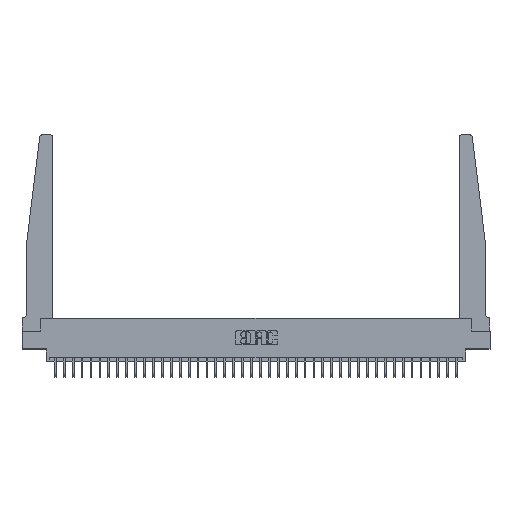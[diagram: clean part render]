
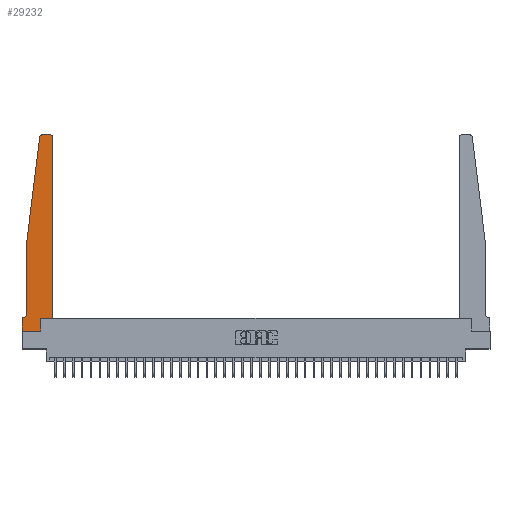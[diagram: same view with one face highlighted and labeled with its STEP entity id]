
A CAD part, top view. The second image highlights one B-rep face of the part: STEP entity #29232.
In plain terms, the highlighted planar face has unit normal (0, 0, 1).
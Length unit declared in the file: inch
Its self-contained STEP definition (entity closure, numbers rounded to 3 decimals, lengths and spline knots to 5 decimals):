
#158 = VECTOR ( 'NONE', #11250, 39.37008 ) ;
#385 = LINE ( 'NONE', #22990, #17930 ) ;
#425 = VERTEX_POINT ( 'NONE', #16666 ) ;
#760 = DIRECTION ( 'NONE',  ( 1., 0., 0. ) ) ;
#777 = CARTESIAN_POINT ( 'NONE',  ( 0.27653, 2.75, 0.37 ) ) ;
#1232 = CARTESIAN_POINT ( 'NONE',  ( 0.425, 2.72, 0.37 ) ) ;
#1611 = DIRECTION ( 'NONE',  ( -1., 0., 0. ) ) ;
#2733 = LINE ( 'NONE', #17054, #158 ) ;
#2762 = VERTEX_POINT ( 'NONE', #23885 ) ;
#2818 = VERTEX_POINT ( 'NONE', #35410 ) ;
#3502 = VECTOR ( 'NONE', #29156, 39.37008 ) ;
#5674 = CARTESIAN_POINT ( 'NONE',  ( 0.425, 0.18, 0.37 ) ) ;
#5698 = CIRCLE ( 'NONE', #6887, 0.05 ) ;
#6228 = EDGE_CURVE ( 'NONE', #24817, #22424, #14608, .T. ) ;
#6242 = EDGE_CURVE ( 'NONE', #9802, #425, #25441, .T. ) ;
#6554 = CARTESIAN_POINT ( 'NONE',  ( 0.25, 2.75, 0.37 ) ) ;
#6887 = AXIS2_PLACEMENT_3D ( 'NONE', #10128, #27002, #1611 ) ;
#7701 = CIRCLE ( 'NONE', #30194, 0.03 ) ;
#7858 = CARTESIAN_POINT ( 'NONE',  ( 0.065, 1.25, 0.37 ) ) ;
#8149 = CARTESIAN_POINT ( 'NONE',  ( 0.2605, 0.18, 0.37 ) ) ;
#8686 = DIRECTION ( 'NONE',  ( 0., 0., 1. ) ) ;
#8942 = ORIENTED_EDGE ( 'NONE', *, *, #28609, .T. ) ;
#9554 = EDGE_CURVE ( 'NONE', #26657, #9802, #35755, .T. ) ;
#9802 = VERTEX_POINT ( 'NONE', #22740 ) ;
#10128 = CARTESIAN_POINT ( 'NONE',  ( 0.015, 0.2375, 0.37 ) ) ;
#11250 = DIRECTION ( 'NONE',  ( 1., 0., 0. ) ) ;
#11584 = EDGE_CURVE ( 'NONE', #14837, #26657, #5698, .T. ) ;
#11778 = DIRECTION ( 'NONE',  ( 0., 1., 0. ) ) ;
#12047 = ORIENTED_EDGE ( 'NONE', *, *, #30227, .T. ) ;
#12601 = EDGE_CURVE ( 'NONE', #25482, #14789, #22620, .T. ) ;
#13620 = CARTESIAN_POINT ( 'NONE',  ( 0.065, 0.2375, 0.37 ) ) ;
#13943 = DIRECTION ( 'NONE',  ( 0., 0., 1. ) ) ;
#14157 = CARTESIAN_POINT ( 'NONE',  ( 0., 0., 0.37 ) ) ;
#14608 = CIRCLE ( 'NONE', #29384, 0.03 ) ;
#14747 = LINE ( 'NONE', #5674, #16177 ) ;
#14789 = VERTEX_POINT ( 'NONE', #7858 ) ;
#14837 = VERTEX_POINT ( 'NONE', #13620 ) ;
#14908 = VECTOR ( 'NONE', #34289, 39.37008 ) ;
#15116 = CARTESIAN_POINT ( 'NONE',  ( 0.395, 2.72, 0.37 ) ) ;
#15720 = CARTESIAN_POINT ( 'NONE',  ( 0.065, 0.1875, 0.37 ) ) ;
#16177 = VECTOR ( 'NONE', #11778, 39.37008 ) ;
#16666 = CARTESIAN_POINT ( 'NONE',  ( 0., 0., 0.37 ) ) ;
#17054 = CARTESIAN_POINT ( 'NONE',  ( 0.425, 0.18, 0.37 ) ) ;
#17352 = EDGE_CURVE ( 'NONE', #22424, #32955, #20651, .T. ) ;
#17930 = VECTOR ( 'NONE', #760, 39.37008 ) ;
#18146 = EDGE_CURVE ( 'NONE', #32955, #25482, #7701, .T. ) ;
#18653 = EDGE_CURVE ( 'NONE', #14789, #14837, #35620, .T. ) ;
#19149 = ORIENTED_EDGE ( 'NONE', *, *, #28237, .T. ) ;
#19338 = CARTESIAN_POINT ( 'NONE',  ( 0.015, 0.1875, 0.37 ) ) ;
#19689 = PLANE ( 'NONE',  #28530 ) ;
#19866 = FACE_OUTER_BOUND ( 'NONE', #34599, .T. ) ;
#20321 = DIRECTION ( 'NONE',  ( 0., 0., 1. ) ) ;
#20559 = CARTESIAN_POINT ( 'NONE',  ( 0.27653, 2.72, 0.37 ) ) ;
#20651 = LINE ( 'NONE', #6554, #3502 ) ;
#21343 = ORIENTED_EDGE ( 'NONE', *, *, #22675, .T. ) ;
#21644 = VECTOR ( 'NONE', #36125, 39.37008 ) ;
#22424 = VERTEX_POINT ( 'NONE', #32023 ) ;
#22620 = LINE ( 'NONE', #36549, #28788 ) ;
#22675 = EDGE_CURVE ( 'NONE', #2762, #24817, #14747, .T. ) ;
#22740 = CARTESIAN_POINT ( 'NONE',  ( 0., 0.1875, 0.37 ) ) ;
#22990 = CARTESIAN_POINT ( 'NONE',  ( 0., 0., 0.37 ) ) ;
#23885 = CARTESIAN_POINT ( 'NONE',  ( 0.425, 0.18, 0.37 ) ) ;
#24817 = VERTEX_POINT ( 'NONE', #1232 ) ;
#25373 = DIRECTION ( 'NONE',  ( 1., 0., 0. ) ) ;
#25441 = LINE ( 'NONE', #14157, #35340 ) ;
#25482 = VERTEX_POINT ( 'NONE', #32091 ) ;
#25725 = LINE ( 'NONE', #34093, #14908 ) ;
#26341 = CARTESIAN_POINT ( 'NONE',  ( 0.065, 1.25, 0.37 ) ) ;
#26657 = VERTEX_POINT ( 'NONE', #19338 ) ;
#27002 = DIRECTION ( 'NONE',  ( 0., 0., -1. ) ) ;
#27085 = DIRECTION ( 'NONE',  ( 0., -1., 0. ) ) ;
#27713 = ORIENTED_EDGE ( 'NONE', *, *, #18146, .T. ) ;
#28237 = EDGE_CURVE ( 'NONE', #425, #2818, #385, .T. ) ;
#28394 = CARTESIAN_POINT ( 'NONE',  ( 0., 0.1875, 0.37 ) ) ;
#28530 = AXIS2_PLACEMENT_3D ( 'NONE', #28394, #13943, #36565 ) ;
#28609 = EDGE_CURVE ( 'NONE', #2818, #29728, #25725, .T. ) ;
#28788 = VECTOR ( 'NONE', #33948, 39.37008 ) ;
#28957 = ORIENTED_EDGE ( 'NONE', *, *, #17352, .T. ) ;
#29057 = ORIENTED_EDGE ( 'NONE', *, *, #6242, .T. ) ;
#29061 = ORIENTED_EDGE ( 'NONE', *, *, #6228, .T. ) ;
#29156 = DIRECTION ( 'NONE',  ( -1., 0., 0. ) ) ;
#29232 = ADVANCED_FACE ( 'NONE', ( #19866 ), #19689, .T. ) ;
#29384 = AXIS2_PLACEMENT_3D ( 'NONE', #15116, #20321, #34798 ) ;
#29534 = ORIENTED_EDGE ( 'NONE', *, *, #12601, .T. ) ;
#29728 = VERTEX_POINT ( 'NONE', #8149 ) ;
#30194 = AXIS2_PLACEMENT_3D ( 'NONE', #20559, #8686, #25373 ) ;
#30220 = VECTOR ( 'NONE', #27085, 39.37008 ) ;
#30227 = EDGE_CURVE ( 'NONE', #29728, #2762, #2733, .T. ) ;
#31555 = DIRECTION ( 'NONE',  ( 0., -1., 0. ) ) ;
#31923 = ORIENTED_EDGE ( 'NONE', *, *, #9554, .T. ) ;
#32023 = CARTESIAN_POINT ( 'NONE',  ( 0.395, 2.75, 0.37 ) ) ;
#32091 = CARTESIAN_POINT ( 'NONE',  ( 0.24675, 2.72367, 0.37 ) ) ;
#32870 = ORIENTED_EDGE ( 'NONE', *, *, #18653, .T. ) ;
#32955 = VERTEX_POINT ( 'NONE', #777 ) ;
#33948 = DIRECTION ( 'NONE',  ( -0.122, -0.992, 0. ) ) ;
#34093 = CARTESIAN_POINT ( 'NONE',  ( 0.2605, 0.18, 0.37 ) ) ;
#34289 = DIRECTION ( 'NONE',  ( 0., 1., 0. ) ) ;
#34599 = EDGE_LOOP ( 'NONE', ( #28957, #27713, #29534, #32870, #35727, #31923, #29057, #19149, #8942, #12047, #21343, #29061 ) ) ;
#34798 = DIRECTION ( 'NONE',  ( 1., 0., 0. ) ) ;
#35340 = VECTOR ( 'NONE', #31555, 39.37008 ) ;
#35410 = CARTESIAN_POINT ( 'NONE',  ( 0.2605, 0., 0.37 ) ) ;
#35620 = LINE ( 'NONE', #26341, #30220 ) ;
#35727 = ORIENTED_EDGE ( 'NONE', *, *, #11584, .T. ) ;
#35755 = LINE ( 'NONE', #15720, #21644 ) ;
#36125 = DIRECTION ( 'NONE',  ( -1., 0., 0. ) ) ;
#36549 = CARTESIAN_POINT ( 'NONE',  ( 0.065, 1.25, 0.37 ) ) ;
#36565 = DIRECTION ( 'NONE',  ( 1., 0., 0. ) ) ;
